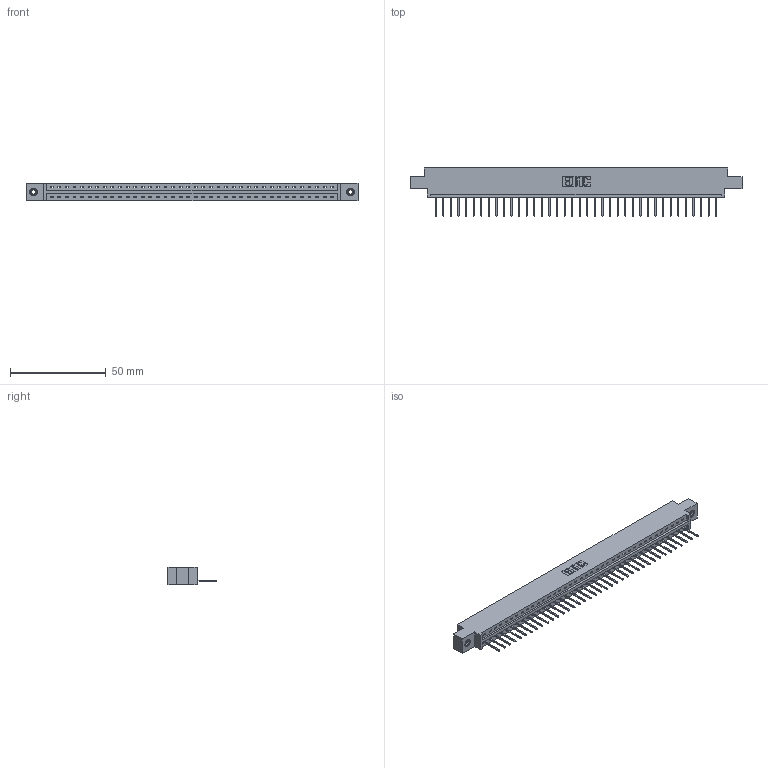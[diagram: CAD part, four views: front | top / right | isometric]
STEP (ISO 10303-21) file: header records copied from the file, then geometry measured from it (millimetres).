
FILE_DESCRIPTION (( 'STEP AP203' ), '1' );
FILE_NAME ('837-038-523-608.STEP', '2021-08-04T14:45:40', ( '' ), ( '' ), 'SwSTEP 2.0', 'SolidWorks 2020', '' );
FILE_SCHEMA (( 'CONFIG_CONTROL_DESIGN' ));
Length unit declared in the file: inch
Products named in the file (4): 837-038-523-608; 345-250-001_345-250-003-102; 837 Part_0.170 Offset - 0.156 Dia-TI; 345-292-001_345-293-123
Assembly tree (41 placements, depth 2):
  837-038-523-608
    837 Part_0.170 Offset - 0.156 Dia-TI
    345-292-001_345-293-123  x38
    345-250-001_345-250-003-102  x2
Bounding box: 173.58 x 25.15 x 9.4 mm (x, y, z)
Volume: 17852.3 mm3; surface area: 18585.2 mm2
Topology: 41 solids, 41 shells, 2534 faces, 7603 edges, 5010 vertices
Faces by surface type: plane 1854, cylinder 664, cone 12, torus 4
Entity records: 30100 total; most frequent: CARTESIAN_POINT 5223, ORIENTED_EDGE 5190, DIRECTION 4437, EDGE_CURVE 2595, LINE 2447, VECTOR 2447, VERTEX_POINT 1724, AXIS2_PLACEMENT_3D 995
